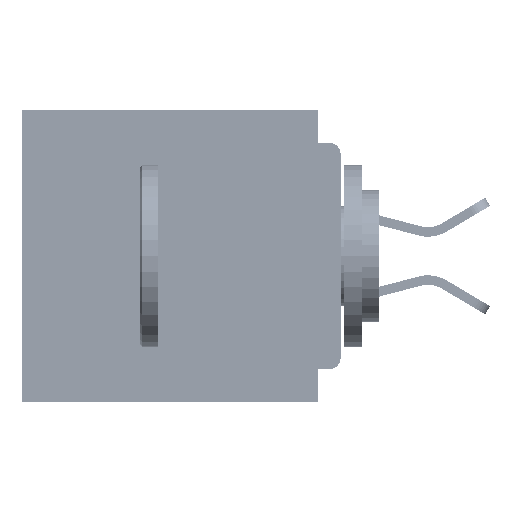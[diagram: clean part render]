
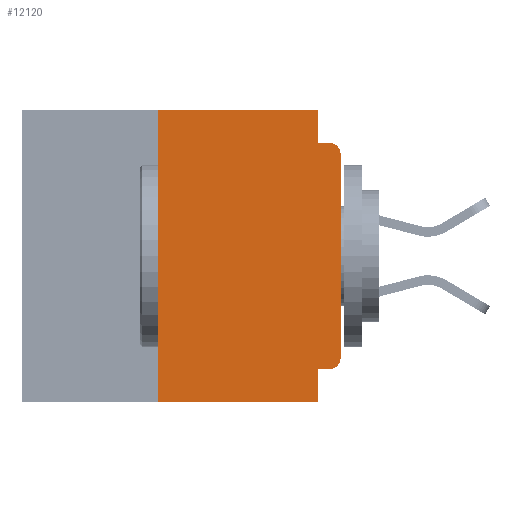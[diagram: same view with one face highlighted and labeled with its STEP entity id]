
A CAD part, left-side view. The second image highlights one B-rep face of the part: STEP entity #12120.
In plain terms, the highlighted planar face has unit normal (-1, 0, 0).
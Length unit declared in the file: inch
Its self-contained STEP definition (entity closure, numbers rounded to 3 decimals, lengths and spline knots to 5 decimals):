
#1361 = VERTEX_POINT ( 'NONE', #12879 ) ;
#1445 = CARTESIAN_POINT ( 'NONE',  ( 0., 0., -0.355 ) ) ;
#1550 = ORIENTED_EDGE ( 'NONE', *, *, #10802, .F. ) ;
#1726 = DIRECTION ( 'NONE',  ( 1., 0., 0. ) ) ;
#2009 = VECTOR ( 'NONE', #2525, 39.37008 ) ;
#2525 = DIRECTION ( 'NONE',  ( 0., 0., -1. ) ) ;
#2555 = DIRECTION ( 'NONE',  ( 0., 0., 1. ) ) ;
#5195 = CARTESIAN_POINT ( 'NONE',  ( 0., 0.25, -0.4 ) ) ;
#5828 = DIRECTION ( 'NONE',  ( 0., 1., 0. ) ) ;
#6196 = CARTESIAN_POINT ( 'NONE',  ( 0., 0., -0.06 ) ) ;
#6656 = EDGE_CURVE ( 'NONE', #49707, #7669, #34876, .T. ) ;
#6827 = VERTEX_POINT ( 'NONE', #41522 ) ;
#6904 = EDGE_CURVE ( 'NONE', #35257, #47826, #20071, .T. ) ;
#6944 = LINE ( 'NONE', #27448, #28434 ) ;
#7112 = ORIENTED_EDGE ( 'NONE', *, *, #27529, .F. ) ;
#7669 = VERTEX_POINT ( 'NONE', #16736 ) ;
#9285 = AXIS2_PLACEMENT_3D ( 'NONE', #24482, #54384, #28820 ) ;
#10281 = DIRECTION ( 'NONE',  ( 0., -1., 0. ) ) ;
#10802 = EDGE_CURVE ( 'NONE', #33676, #51643, #6944, .T. ) ;
#11992 = LINE ( 'NONE', #32656, #33444 ) ;
#12120 = ADVANCED_FACE ( 'NONE', ( #40995 ), #23180, .F. ) ;
#12829 = EDGE_LOOP ( 'NONE', ( #40727, #44114, #1550, #15752, #18967, #31373, #43808, #47412, #7112, #44092 ) ) ;
#12879 = CARTESIAN_POINT ( 'NONE',  ( 0., 0.015, -0.355 ) ) ;
#13382 = VECTOR ( 'NONE', #23971, 39.37008 ) ;
#13560 = LINE ( 'NONE', #1445, #45009 ) ;
#13738 = CARTESIAN_POINT ( 'NONE',  ( 0., 0., -0.34 ) ) ;
#13796 = EDGE_CURVE ( 'NONE', #49707, #35257, #19338, .T. ) ;
#14070 = CIRCLE ( 'NONE', #9285, 0.015 ) ;
#14114 = EDGE_CURVE ( 'NONE', #1361, #24752, #14070, .T. ) ;
#14589 = CARTESIAN_POINT ( 'NONE',  ( 0., 0.437, -0.4 ) ) ;
#15752 = ORIENTED_EDGE ( 'NONE', *, *, #21889, .F. ) ;
#16668 = CARTESIAN_POINT ( 'NONE',  ( 0., 0.25, 0. ) ) ;
#16736 = CARTESIAN_POINT ( 'NONE',  ( 0., 0.031, -0.4 ) ) ;
#17487 = CARTESIAN_POINT ( 'NONE',  ( 0., 0.25, -0.4 ) ) ;
#18509 = CARTESIAN_POINT ( 'NONE',  ( 0., 0.015, -0.06 ) ) ;
#18967 = ORIENTED_EDGE ( 'NONE', *, *, #6904, .F. ) ;
#19338 = LINE ( 'NONE', #5195, #40779 ) ;
#19600 = AXIS2_PLACEMENT_3D ( 'NONE', #53096, #1726, #31837 ) ;
#19687 = CARTESIAN_POINT ( 'NONE',  ( 0., 0.031, -0.4 ) ) ;
#20071 = LINE ( 'NONE', #42076, #31484 ) ;
#20538 = DIRECTION ( 'NONE',  ( 0., -1., 0. ) ) ;
#21889 = EDGE_CURVE ( 'NONE', #47826, #33676, #27588, .T. ) ;
#22112 = VECTOR ( 'NONE', #10281, 39.37008 ) ;
#22794 = DIRECTION ( 'NONE',  ( 0., 0., -1. ) ) ;
#23180 = PLANE ( 'NONE',  #19600 ) ;
#23971 = DIRECTION ( 'NONE',  ( 0., 0., -1. ) ) ;
#24482 = CARTESIAN_POINT ( 'NONE',  ( 0., 0.015, -0.34 ) ) ;
#24752 = VERTEX_POINT ( 'NONE', #13738 ) ;
#25223 = CIRCLE ( 'NONE', #43525, 0.015 ) ;
#27448 = CARTESIAN_POINT ( 'NONE',  ( 0., 0., -0.045 ) ) ;
#27529 = EDGE_CURVE ( 'NONE', #1361, #6827, #13560, .T. ) ;
#27588 = LINE ( 'NONE', #28299, #2009 ) ;
#27965 = CARTESIAN_POINT ( 'NONE',  ( 0., 0.031, -0.045 ) ) ;
#28299 = CARTESIAN_POINT ( 'NONE',  ( 0., 0.031, 0. ) ) ;
#28434 = VECTOR ( 'NONE', #48781, 39.37008 ) ;
#28820 = DIRECTION ( 'NONE',  ( 0., 0., -1. ) ) ;
#29640 = VERTEX_POINT ( 'NONE', #6196 ) ;
#30235 = EDGE_CURVE ( 'NONE', #6827, #7669, #36120, .T. ) ;
#31070 = CARTESIAN_POINT ( 'NONE',  ( 0., 0.031, 0. ) ) ;
#31373 = ORIENTED_EDGE ( 'NONE', *, *, #13796, .F. ) ;
#31484 = VECTOR ( 'NONE', #20538, 39.37008 ) ;
#31837 = DIRECTION ( 'NONE',  ( 0., 0., -1. ) ) ;
#32656 = CARTESIAN_POINT ( 'NONE',  ( 0., 0., 0. ) ) ;
#33444 = VECTOR ( 'NONE', #2555, 39.37008 ) ;
#33676 = VERTEX_POINT ( 'NONE', #27965 ) ;
#34876 = LINE ( 'NONE', #14589, #22112 ) ;
#35257 = VERTEX_POINT ( 'NONE', #16668 ) ;
#36120 = LINE ( 'NONE', #19687, #13382 ) ;
#36848 = CARTESIAN_POINT ( 'NONE',  ( 0., 0.015, -0.045 ) ) ;
#40727 = ORIENTED_EDGE ( 'NONE', *, *, #55408, .T. ) ;
#40779 = VECTOR ( 'NONE', #52199, 39.37008 ) ;
#40995 = FACE_OUTER_BOUND ( 'NONE', #12829, .T. ) ;
#41522 = CARTESIAN_POINT ( 'NONE',  ( 0., 0.031, -0.355 ) ) ;
#42076 = CARTESIAN_POINT ( 'NONE',  ( 0., 0.437, 0. ) ) ;
#43525 = AXIS2_PLACEMENT_3D ( 'NONE', #18509, #48439, #22794 ) ;
#43808 = ORIENTED_EDGE ( 'NONE', *, *, #6656, .T. ) ;
#44092 = ORIENTED_EDGE ( 'NONE', *, *, #14114, .T. ) ;
#44114 = ORIENTED_EDGE ( 'NONE', *, *, #51462, .T. ) ;
#45009 = VECTOR ( 'NONE', #5828, 39.37008 ) ;
#47412 = ORIENTED_EDGE ( 'NONE', *, *, #30235, .F. ) ;
#47826 = VERTEX_POINT ( 'NONE', #31070 ) ;
#48439 = DIRECTION ( 'NONE',  ( -1., 0., 0. ) ) ;
#48781 = DIRECTION ( 'NONE',  ( 0., -1., 0. ) ) ;
#49707 = VERTEX_POINT ( 'NONE', #17487 ) ;
#51462 = EDGE_CURVE ( 'NONE', #29640, #51643, #25223, .T. ) ;
#51643 = VERTEX_POINT ( 'NONE', #36848 ) ;
#52199 = DIRECTION ( 'NONE',  ( 0., 0., 1. ) ) ;
#53096 = CARTESIAN_POINT ( 'NONE',  ( 0., 0.437, 0. ) ) ;
#54384 = DIRECTION ( 'NONE',  ( -1., 0., 0. ) ) ;
#55408 = EDGE_CURVE ( 'NONE', #24752, #29640, #11992, .T. ) ;
